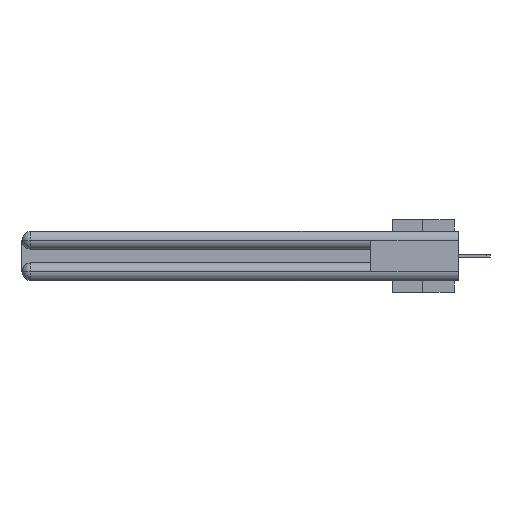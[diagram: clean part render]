
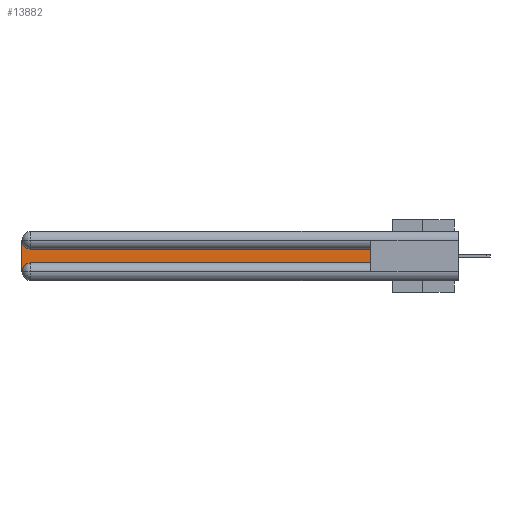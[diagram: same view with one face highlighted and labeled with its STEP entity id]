
A CAD part, left-side view. The second image highlights one B-rep face of the part: STEP entity #13882.
In plain terms, the highlighted planar face has unit normal (-1, 0, 0).
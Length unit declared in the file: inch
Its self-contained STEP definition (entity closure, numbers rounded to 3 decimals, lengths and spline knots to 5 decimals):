
#2816 = CARTESIAN_POINT ( 'NONE',  ( 0.075, 2.94, -0.2175 ) ) ;
#3946 = DIRECTION ( 'NONE',  ( 0., 0., -1. ) ) ;
#4751 = CARTESIAN_POINT ( 'NONE',  ( 0.075, 3., -0.2775 ) ) ;
#4957 = VECTOR ( 'NONE', #3946, 39.37008 ) ;
#6340 = EDGE_LOOP ( 'NONE', ( #26634, #38223, #20688, #13730, #21470, #29419 ) ) ;
#7385 = EDGE_CURVE ( 'NONE', #11387, #36213, #21893, .T. ) ;
#8823 = CARTESIAN_POINT ( 'NONE',  ( 0.075, 2.94, -0.0625 ) ) ;
#9090 = VERTEX_POINT ( 'NONE', #21073 ) ;
#9191 = PLANE ( 'NONE',  #16562 ) ;
#9712 = VERTEX_POINT ( 'NONE', #38474 ) ;
#11387 = VERTEX_POINT ( 'NONE', #27103 ) ;
#12023 = CARTESIAN_POINT ( 'NONE',  ( 0.075, 2.94, -0.2775 ) ) ;
#12445 = VECTOR ( 'NONE', #27871, 39.37008 ) ;
#12964 = CARTESIAN_POINT ( 'NONE',  ( 0.075, 3., -0.1225 ) ) ;
#13730 = ORIENTED_EDGE ( 'NONE', *, *, #19927, .T. ) ;
#13882 = ADVANCED_FACE ( 'NONE', ( #18359 ), #9191, .F. ) ;
#16390 = CARTESIAN_POINT ( 'NONE',  ( 0.075, 0.6, -0.2175 ) ) ;
#16527 = EDGE_CURVE ( 'NONE', #9712, #11387, #24952, .T. ) ;
#16562 = AXIS2_PLACEMENT_3D ( 'NONE', #12964, #25124, #30895 ) ;
#17590 = DIRECTION ( 'NONE',  ( 0., 0., -1. ) ) ;
#18121 = CARTESIAN_POINT ( 'NONE',  ( 0.075, 0.6, -0.1225 ) ) ;
#18359 = FACE_OUTER_BOUND ( 'NONE', #6340, .T. ) ;
#18593 = EDGE_CURVE ( 'NONE', #36213, #9090, #29450, .T. ) ;
#19927 = EDGE_CURVE ( 'NONE', #35424, #20103, #31421, .T. ) ;
#19969 = AXIS2_PLACEMENT_3D ( 'NONE', #12023, #21381, #24178 ) ;
#20103 = VERTEX_POINT ( 'NONE', #2816 ) ;
#20121 = DIRECTION ( 'NONE',  ( 0., -1., 0. ) ) ;
#20688 = ORIENTED_EDGE ( 'NONE', *, *, #23680, .T. ) ;
#21073 = CARTESIAN_POINT ( 'NONE',  ( 0.075, 3., -0.0625 ) ) ;
#21381 = DIRECTION ( 'NONE',  ( 1., 0., 0. ) ) ;
#21470 = ORIENTED_EDGE ( 'NONE', *, *, #28153, .T. ) ;
#21893 = LINE ( 'NONE', #18121, #12445 ) ;
#22443 = CARTESIAN_POINT ( 'NONE',  ( 0.075, 3., -0.2175 ) ) ;
#22465 = AXIS2_PLACEMENT_3D ( 'NONE', #8823, #33313, #17590 ) ;
#23295 = LINE ( 'NONE', #35454, #24303 ) ;
#23680 = EDGE_CURVE ( 'NONE', #9090, #35424, #37607, .T. ) ;
#24178 = DIRECTION ( 'NONE',  ( 0., 0., -1. ) ) ;
#24303 = VECTOR ( 'NONE', #20121, 39.37008 ) ;
#24952 = LINE ( 'NONE', #16390, #33981 ) ;
#25124 = DIRECTION ( 'NONE',  ( 1., 0., 0. ) ) ;
#26634 = ORIENTED_EDGE ( 'NONE', *, *, #7385, .T. ) ;
#27103 = CARTESIAN_POINT ( 'NONE',  ( 0.075, 0.6, -0.1225 ) ) ;
#27871 = DIRECTION ( 'NONE',  ( 0., 1., 0. ) ) ;
#27978 = CARTESIAN_POINT ( 'NONE',  ( 0.075, 2.94, -0.1225 ) ) ;
#28153 = EDGE_CURVE ( 'NONE', #20103, #9712, #23295, .T. ) ;
#29419 = ORIENTED_EDGE ( 'NONE', *, *, #16527, .T. ) ;
#29450 = CIRCLE ( 'NONE', #22465, 0.06 ) ;
#30895 = DIRECTION ( 'NONE',  ( 0., 0., -1. ) ) ;
#31421 = CIRCLE ( 'NONE', #19969, 0.06 ) ;
#33313 = DIRECTION ( 'NONE',  ( 1., 0., 0. ) ) ;
#33981 = VECTOR ( 'NONE', #34911, 39.37008 ) ;
#34911 = DIRECTION ( 'NONE',  ( 0., 0., 1. ) ) ;
#35424 = VERTEX_POINT ( 'NONE', #4751 ) ;
#35454 = CARTESIAN_POINT ( 'NONE',  ( 0.075, 0.6, -0.2175 ) ) ;
#36213 = VERTEX_POINT ( 'NONE', #27978 ) ;
#37607 = LINE ( 'NONE', #22443, #4957 ) ;
#38223 = ORIENTED_EDGE ( 'NONE', *, *, #18593, .T. ) ;
#38474 = CARTESIAN_POINT ( 'NONE',  ( 0.075, 0.6, -0.2175 ) ) ;
